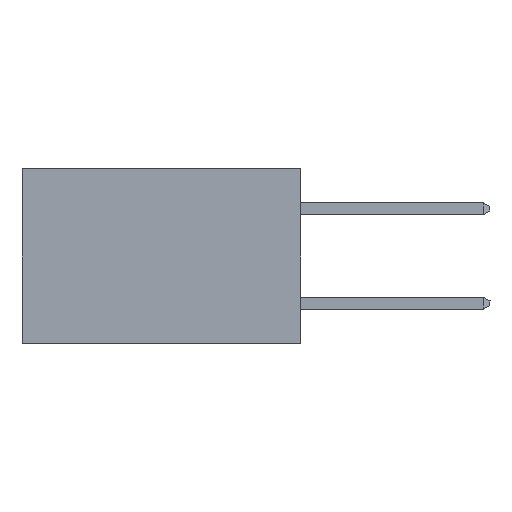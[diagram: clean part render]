
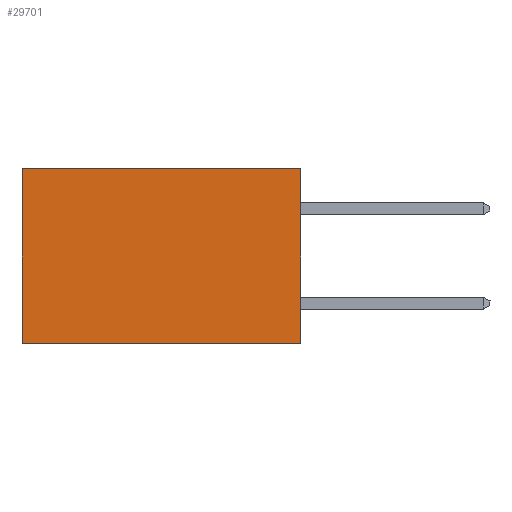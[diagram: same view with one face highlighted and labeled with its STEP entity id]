
A CAD part, left-side view. The second image highlights one B-rep face of the part: STEP entity #29701.
In plain terms, the highlighted planar face has unit normal (-1, 0, 0).
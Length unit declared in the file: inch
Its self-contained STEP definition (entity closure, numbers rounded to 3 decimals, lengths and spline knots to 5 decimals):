
#1153 = VERTEX_POINT ( 'NONE', #11208 ) ;
#2522 = DIRECTION ( 'NONE',  ( 0., 1., 0. ) ) ;
#2561 = CARTESIAN_POINT ( 'NONE',  ( 0.277, 0., 0. ) ) ;
#2667 = FACE_OUTER_BOUND ( 'NONE', #8590, .T. ) ;
#3497 = ORIENTED_EDGE ( 'NONE', *, *, #33351, .F. ) ;
#7455 = VERTEX_POINT ( 'NONE', #18516 ) ;
#8373 = ORIENTED_EDGE ( 'NONE', *, *, #26333, .F. ) ;
#8478 = VECTOR ( 'NONE', #33191, 39.37008 ) ;
#8590 = EDGE_LOOP ( 'NONE', ( #22407, #8373, #3497, #28728 ) ) ;
#8627 = DIRECTION ( 'NONE',  ( 0., 1., 0. ) ) ;
#9840 = EDGE_CURVE ( 'NONE', #19752, #7455, #9994, .T. ) ;
#9994 = LINE ( 'NONE', #19228, #17779 ) ;
#10356 = CARTESIAN_POINT ( 'NONE',  ( 0.277, 0., -0.37 ) ) ;
#11208 = CARTESIAN_POINT ( 'NONE',  ( 0.277, 0., -0.37 ) ) ;
#11312 = CARTESIAN_POINT ( 'NONE',  ( 0.277, 0., -0.37 ) ) ;
#12365 = LINE ( 'NONE', #11312, #14002 ) ;
#12781 = CARTESIAN_POINT ( 'NONE',  ( 0.277, 0.59, 0. ) ) ;
#13357 = EDGE_CURVE ( 'NONE', #22504, #19752, #32652, .T. ) ;
#14002 = VECTOR ( 'NONE', #8627, 39.37008 ) ;
#15039 = CARTESIAN_POINT ( 'NONE',  ( 0.277, 0., -0.37 ) ) ;
#15603 = DIRECTION ( 'NONE',  ( 1., 0., 0. ) ) ;
#17779 = VECTOR ( 'NONE', #19846, 39.37008 ) ;
#18516 = CARTESIAN_POINT ( 'NONE',  ( 0.277, 0.59, -0.37 ) ) ;
#19228 = CARTESIAN_POINT ( 'NONE',  ( 0.277, 0.59, -0.37 ) ) ;
#19752 = VERTEX_POINT ( 'NONE', #12781 ) ;
#19846 = DIRECTION ( 'NONE',  ( 0., 0., -1. ) ) ;
#20809 = LINE ( 'NONE', #15039, #8478 ) ;
#21080 = AXIS2_PLACEMENT_3D ( 'NONE', #10356, #15603, #33758 ) ;
#22407 = ORIENTED_EDGE ( 'NONE', *, *, #9840, .T. ) ;
#22504 = VERTEX_POINT ( 'NONE', #29477 ) ;
#26058 = PLANE ( 'NONE',  #21080 ) ;
#26333 = EDGE_CURVE ( 'NONE', #1153, #7455, #12365, .T. ) ;
#28728 = ORIENTED_EDGE ( 'NONE', *, *, #13357, .T. ) ;
#29477 = CARTESIAN_POINT ( 'NONE',  ( 0.277, 0., 0. ) ) ;
#29701 = ADVANCED_FACE ( 'NONE', ( #2667 ), #26058, .F. ) ;
#31884 = VECTOR ( 'NONE', #2522, 39.37008 ) ;
#32652 = LINE ( 'NONE', #2561, #31884 ) ;
#33191 = DIRECTION ( 'NONE',  ( 0., 0., -1. ) ) ;
#33351 = EDGE_CURVE ( 'NONE', #22504, #1153, #20809, .T. ) ;
#33758 = DIRECTION ( 'NONE',  ( 0., 0., -1. ) ) ;
